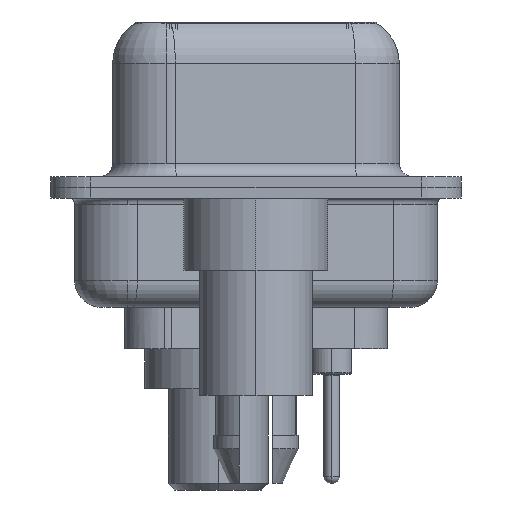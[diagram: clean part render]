
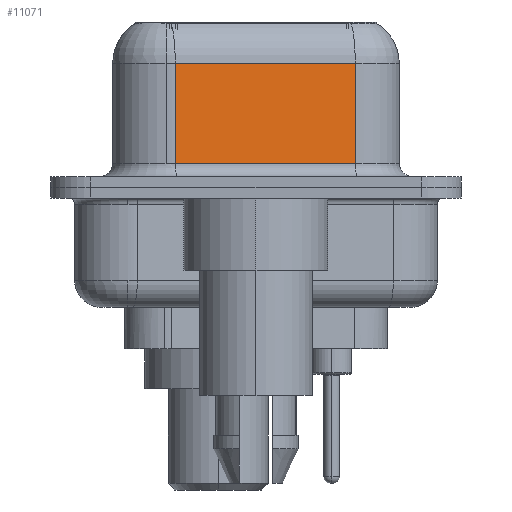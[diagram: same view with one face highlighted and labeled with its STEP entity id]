
A CAD part, left-side view. The second image highlights one B-rep face of the part: STEP entity #11071.
In plain terms, the highlighted planar face has unit normal (-0.985, -0.174, 0).
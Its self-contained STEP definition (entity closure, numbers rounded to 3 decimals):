
#161 = ORIENTED_EDGE ( 'NONE', *, *, #17000, .T. ) ;
#1109 = VECTOR ( 'NONE', #21955, 1000. ) ;
#1219 = CARTESIAN_POINT ( 'NONE',  ( 5.621, -3.722, 4.65 ) ) ;
#1735 = AXIS2_PLACEMENT_3D ( 'NONE', #34761, #10483, #13239 ) ;
#2041 = CARTESIAN_POINT ( 'NONE',  ( 5.621, -3.722, 4.65 ) ) ;
#2436 = FACE_OUTER_BOUND ( 'NONE', #24912, .T. ) ;
#3084 = CARTESIAN_POINT ( 'NONE',  ( 5.621, -3.722, 0.9 ) ) ;
#4533 = CARTESIAN_POINT ( 'NONE',  ( 5.621, -3.722, 6.4 ) ) ;
#4947 = EDGE_CURVE ( 'NONE', #28134, #8718, #34426, .T. ) ;
#5945 = DIRECTION ( 'NONE',  ( 0.174, -0.985, 0. ) ) ;
#6737 = EDGE_CURVE ( 'NONE', #12179, #17041, #29979, .T. ) ;
#8718 = VERTEX_POINT ( 'NONE', #14159 ) ;
#10483 = DIRECTION ( 'NONE',  ( 0.985, 0.174, 0. ) ) ;
#10669 = CARTESIAN_POINT ( 'NONE',  ( 4.43, 3.028, 6.4 ) ) ;
#11071 = ADVANCED_FACE ( 'NONE', ( #2436 ), #18535, .F. ) ;
#11208 = VECTOR ( 'NONE', #18164, 1000. ) ;
#11316 = CARTESIAN_POINT ( 'NONE',  ( 5.621, -3.722, 0.9 ) ) ;
#11585 = VECTOR ( 'NONE', #5945, 1000. ) ;
#12179 = VERTEX_POINT ( 'NONE', #14437 ) ;
#13239 = DIRECTION ( 'NONE',  ( -0.174, 0.985, 0. ) ) ;
#14159 = CARTESIAN_POINT ( 'NONE',  ( 4.43, 3.028, 4.65 ) ) ;
#14437 = CARTESIAN_POINT ( 'NONE',  ( 4.43, 3.028, 0.9 ) ) ;
#17000 = EDGE_CURVE ( 'NONE', #8718, #12179, #29295, .T. ) ;
#17041 = VERTEX_POINT ( 'NONE', #3084 ) ;
#18164 = DIRECTION ( 'NONE',  ( 0., 0., -1. ) ) ;
#18535 = PLANE ( 'NONE',  #1735 ) ;
#18957 = ORIENTED_EDGE ( 'NONE', *, *, #4947, .T. ) ;
#19320 = EDGE_CURVE ( 'NONE', #28134, #17041, #27923, .T. ) ;
#21955 = DIRECTION ( 'NONE',  ( 0., 0., -1. ) ) ;
#24912 = EDGE_LOOP ( 'NONE', ( #27941, #18957, #161, #29810 ) ) ;
#26658 = DIRECTION ( 'NONE',  ( -0.174, 0.985, 0. ) ) ;
#27923 = LINE ( 'NONE', #4533, #11208 ) ;
#27941 = ORIENTED_EDGE ( 'NONE', *, *, #19320, .F. ) ;
#28134 = VERTEX_POINT ( 'NONE', #1219 ) ;
#29295 = LINE ( 'NONE', #10669, #1109 ) ;
#29810 = ORIENTED_EDGE ( 'NONE', *, *, #6737, .T. ) ;
#29979 = LINE ( 'NONE', #11316, #11585 ) ;
#33175 = VECTOR ( 'NONE', #26658, 1000. ) ;
#34426 = LINE ( 'NONE', #2041, #33175 ) ;
#34761 = CARTESIAN_POINT ( 'NONE',  ( 5.621, -3.722, 6.4 ) ) ;
